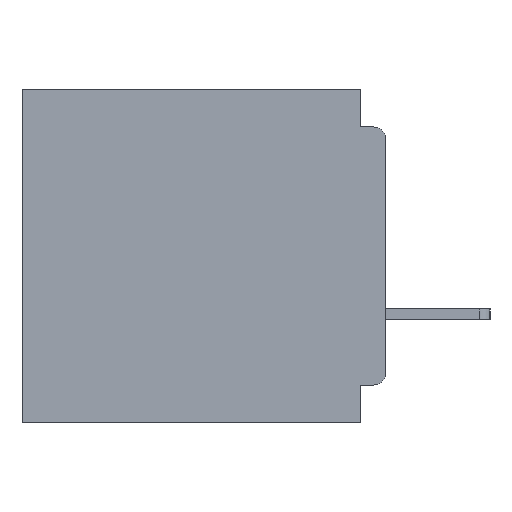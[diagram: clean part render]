
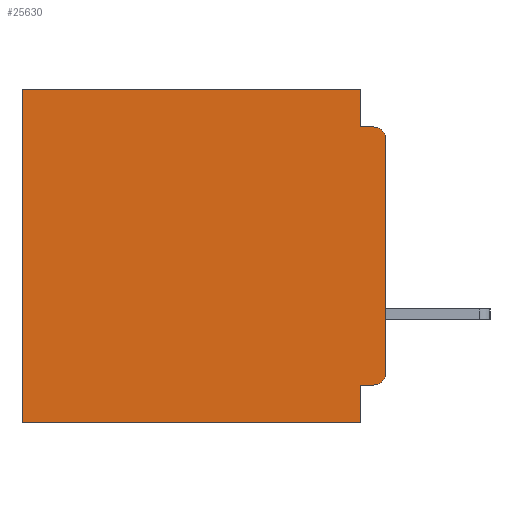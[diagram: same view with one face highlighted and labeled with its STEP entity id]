
A CAD part, left-side view. The second image highlights one B-rep face of the part: STEP entity #25630.
In plain terms, the highlighted planar face has unit normal (-1, 0, 0).
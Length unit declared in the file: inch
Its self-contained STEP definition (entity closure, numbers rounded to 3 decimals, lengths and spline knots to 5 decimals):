
#261 = DIRECTION ( 'NONE',  ( -1., 0., 0. ) ) ;
#727 = VECTOR ( 'NONE', #5699, 39.37008 ) ;
#2024 = CARTESIAN_POINT ( 'NONE',  ( 0.3, 0.031, 0. ) ) ;
#4849 = CARTESIAN_POINT ( 'NONE',  ( 0.3, 0.015, -0.34 ) ) ;
#5170 = CARTESIAN_POINT ( 'NONE',  ( 0.3, 0., -0.4 ) ) ;
#5313 = DIRECTION ( 'NONE',  ( 0., 1., 0. ) ) ;
#5486 = CARTESIAN_POINT ( 'NONE',  ( 0.3, 0.031, -0.045 ) ) ;
#5625 = AXIS2_PLACEMENT_3D ( 'NONE', #4849, #30434, #8516 ) ;
#5699 = DIRECTION ( 'NONE',  ( 0., 0., -1. ) ) ;
#6891 = CARTESIAN_POINT ( 'NONE',  ( 0.3, 0., -0.34 ) ) ;
#7434 = DIRECTION ( 'NONE',  ( 0., 0., -1. ) ) ;
#8516 = DIRECTION ( 'NONE',  ( 0., 0., -1. ) ) ;
#8584 = LINE ( 'NONE', #36938, #36608 ) ;
#8841 = DIRECTION ( 'NONE',  ( 0., 1., 0. ) ) ;
#9497 = CARTESIAN_POINT ( 'NONE',  ( 0.3, 0., -0.045 ) ) ;
#9518 = LINE ( 'NONE', #29513, #26691 ) ;
#9565 = ORIENTED_EDGE ( 'NONE', *, *, #35017, .F. ) ;
#12536 = EDGE_CURVE ( 'NONE', #22166, #20053, #44446, .T. ) ;
#13230 = CARTESIAN_POINT ( 'NONE',  ( 0.3, 0.031, -0.355 ) ) ;
#13544 = EDGE_CURVE ( 'NONE', #28920, #14314, #19349, .T. ) ;
#14314 = VERTEX_POINT ( 'NONE', #33686 ) ;
#14745 = EDGE_CURVE ( 'NONE', #22166, #15230, #9518, .T. ) ;
#15230 = VERTEX_POINT ( 'NONE', #6891 ) ;
#15783 = ORIENTED_EDGE ( 'NONE', *, *, #38805, .T. ) ;
#16427 = EDGE_CURVE ( 'NONE', #26718, #42000, #29936, .T. ) ;
#16810 = VECTOR ( 'NONE', #8841, 39.37008 ) ;
#16818 = DIRECTION ( 'NONE',  ( 0., -1., 0. ) ) ;
#17165 = AXIS2_PLACEMENT_3D ( 'NONE', #36470, #40099, #18248 ) ;
#18248 = DIRECTION ( 'NONE',  ( 0., 0., -1. ) ) ;
#18356 = EDGE_CURVE ( 'NONE', #22987, #15230, #38384, .T. ) ;
#18718 = DIRECTION ( 'NONE',  ( 0., 0., -1. ) ) ;
#19349 = LINE ( 'NONE', #21735, #27987 ) ;
#19505 = VERTEX_POINT ( 'NONE', #40474 ) ;
#19780 = ORIENTED_EDGE ( 'NONE', *, *, #16427, .F. ) ;
#19815 = EDGE_LOOP ( 'NONE', ( #38655, #27816, #32346, #19780, #15783, #37526, #28969, #38108, #9565, #34768 ) ) ;
#20053 = VERTEX_POINT ( 'NONE', #21761 ) ;
#20313 = CARTESIAN_POINT ( 'NONE',  ( 0.3, 0., -0.06 ) ) ;
#21469 = VECTOR ( 'NONE', #5313, 39.37008 ) ;
#21735 = CARTESIAN_POINT ( 'NONE',  ( 0.3, 0.031, -0.4 ) ) ;
#21761 = CARTESIAN_POINT ( 'NONE',  ( 0.3, 0.015, -0.045 ) ) ;
#22166 = VERTEX_POINT ( 'NONE', #20313 ) ;
#22175 = CARTESIAN_POINT ( 'NONE',  ( 0.3, 0.015, -0.06 ) ) ;
#22987 = VERTEX_POINT ( 'NONE', #40164 ) ;
#23189 = VERTEX_POINT ( 'NONE', #26811 ) ;
#23957 = EDGE_CURVE ( 'NONE', #19505, #23189, #8584, .T. ) ;
#25207 = LINE ( 'NONE', #26643, #43328 ) ;
#25630 = ADVANCED_FACE ( 'NONE', ( #39822 ), #32793, .F. ) ;
#25892 = DIRECTION ( 'NONE',  ( 0., 0., -1. ) ) ;
#26643 = CARTESIAN_POINT ( 'NONE',  ( 0.3, 0., 0. ) ) ;
#26691 = VECTOR ( 'NONE', #7434, 39.37008 ) ;
#26718 = VERTEX_POINT ( 'NONE', #46970 ) ;
#26811 = CARTESIAN_POINT ( 'NONE',  ( 0.3, 0.437, -0.4 ) ) ;
#27239 = CARTESIAN_POINT ( 'NONE',  ( 0.3, 0., -0.355 ) ) ;
#27816 = ORIENTED_EDGE ( 'NONE', *, *, #12536, .T. ) ;
#27987 = VECTOR ( 'NONE', #43491, 39.37008 ) ;
#28920 = VERTEX_POINT ( 'NONE', #13230 ) ;
#28969 = ORIENTED_EDGE ( 'NONE', *, *, #44340, .F. ) ;
#29513 = CARTESIAN_POINT ( 'NONE',  ( 0.3, 0., -0.4 ) ) ;
#29936 = LINE ( 'NONE', #2024, #727 ) ;
#30315 = DIRECTION ( 'NONE',  ( 0., 1., 0. ) ) ;
#30434 = DIRECTION ( 'NONE',  ( -1., 0., 0. ) ) ;
#32346 = ORIENTED_EDGE ( 'NONE', *, *, #36533, .F. ) ;
#32793 = PLANE ( 'NONE',  #17165 ) ;
#33686 = CARTESIAN_POINT ( 'NONE',  ( 0.3, 0.031, -0.4 ) ) ;
#34768 = ORIENTED_EDGE ( 'NONE', *, *, #18356, .T. ) ;
#35017 = EDGE_CURVE ( 'NONE', #22987, #28920, #40866, .T. ) ;
#36470 = CARTESIAN_POINT ( 'NONE',  ( 0.3, 0., -0.4 ) ) ;
#36533 = EDGE_CURVE ( 'NONE', #42000, #20053, #46229, .T. ) ;
#36608 = VECTOR ( 'NONE', #18718, 39.37008 ) ;
#36769 = VECTOR ( 'NONE', #16818, 39.37008 ) ;
#36938 = CARTESIAN_POINT ( 'NONE',  ( 0.3, 0.437, -0.4 ) ) ;
#37526 = ORIENTED_EDGE ( 'NONE', *, *, #23957, .T. ) ;
#38108 = ORIENTED_EDGE ( 'NONE', *, *, #13544, .F. ) ;
#38384 = CIRCLE ( 'NONE', #5625, 0.015 ) ;
#38655 = ORIENTED_EDGE ( 'NONE', *, *, #14745, .F. ) ;
#38805 = EDGE_CURVE ( 'NONE', #26718, #19505, #25207, .T. ) ;
#39822 = FACE_OUTER_BOUND ( 'NONE', #19815, .T. ) ;
#40099 = DIRECTION ( 'NONE',  ( 1., 0., 0. ) ) ;
#40164 = CARTESIAN_POINT ( 'NONE',  ( 0.3, 0.015, -0.355 ) ) ;
#40474 = CARTESIAN_POINT ( 'NONE',  ( 0.3, 0.437, 0. ) ) ;
#40866 = LINE ( 'NONE', #27239, #21469 ) ;
#42000 = VERTEX_POINT ( 'NONE', #5486 ) ;
#43328 = VECTOR ( 'NONE', #30315, 39.37008 ) ;
#43491 = DIRECTION ( 'NONE',  ( 0., 0., -1. ) ) ;
#44340 = EDGE_CURVE ( 'NONE', #14314, #23189, #45743, .T. ) ;
#44446 = CIRCLE ( 'NONE', #44874, 0.015 ) ;
#44874 = AXIS2_PLACEMENT_3D ( 'NONE', #22175, #261, #25892 ) ;
#45743 = LINE ( 'NONE', #5170, #16810 ) ;
#46229 = LINE ( 'NONE', #9497, #36769 ) ;
#46970 = CARTESIAN_POINT ( 'NONE',  ( 0.3, 0.031, 0. ) ) ;
